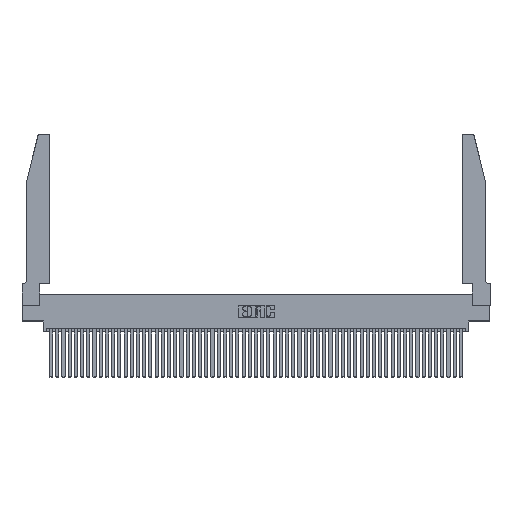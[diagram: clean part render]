
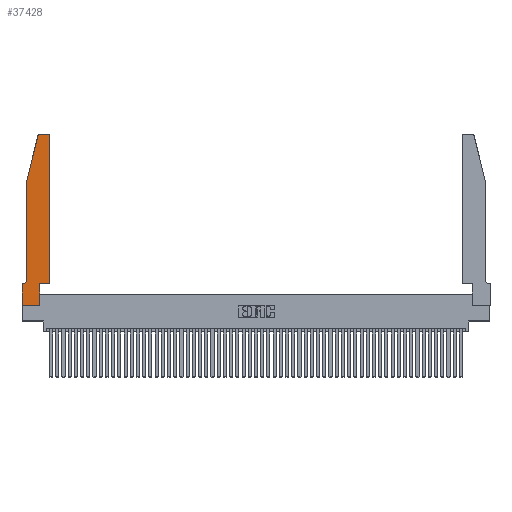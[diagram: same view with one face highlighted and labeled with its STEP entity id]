
A CAD part, top view. The second image highlights one B-rep face of the part: STEP entity #37428.
In plain terms, the highlighted planar face has unit normal (0, 0, 1).
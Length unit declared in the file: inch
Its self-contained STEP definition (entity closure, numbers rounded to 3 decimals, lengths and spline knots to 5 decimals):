
#1467 = VERTEX_POINT ( 'NONE', #30838 ) ;
#4908 = VECTOR ( 'NONE', #38754, 39.37008 ) ;
#5191 = ORIENTED_EDGE ( 'NONE', *, *, #21473, .T. ) ;
#6381 = LINE ( 'NONE', #33834, #38349 ) ;
#10282 = VECTOR ( 'NONE', #19206, 39.37008 ) ;
#10430 = VECTOR ( 'NONE', #53533, 39.37008 ) ;
#10548 = CARTESIAN_POINT ( 'NONE',  ( 0.4205, 2.72, 0.37 ) ) ;
#10825 = CARTESIAN_POINT ( 'NONE',  ( 0.0755, 0.42, 0.37 ) ) ;
#11624 = LINE ( 'NONE', #31659, #10282 ) ;
#11645 = FACE_OUTER_BOUND ( 'NONE', #47028, .T. ) ;
#11831 = ORIENTED_EDGE ( 'NONE', *, *, #52363, .T. ) ;
#12382 = DIRECTION ( 'NONE',  ( 0., 1., 0. ) ) ;
#12933 = VERTEX_POINT ( 'NONE', #28234 ) ;
#13302 = DIRECTION ( 'NONE',  ( 0., -1., 0. ) ) ;
#13652 = LINE ( 'NONE', #20702, #53766 ) ;
#13693 = EDGE_CURVE ( 'NONE', #47984, #1467, #21667, .T. ) ;
#14218 = AXIS2_PLACEMENT_3D ( 'NONE', #49524, #24896, #53677 ) ;
#14464 = CIRCLE ( 'NONE', #14218, 0.03 ) ;
#14589 = CARTESIAN_POINT ( 'NONE',  ( 0.2605, 2.75, 0.37 ) ) ;
#14800 = DIRECTION ( 'NONE',  ( 1., 0., 0. ) ) ;
#15106 = ORIENTED_EDGE ( 'NONE', *, *, #33840, .T. ) ;
#15964 = VECTOR ( 'NONE', #13302, 39.37008 ) ;
#18115 = ORIENTED_EDGE ( 'NONE', *, *, #38437, .T. ) ;
#18135 = CARTESIAN_POINT ( 'NONE',  ( 0.4505, 0.35, 0.37 ) ) ;
#18315 = ORIENTED_EDGE ( 'NONE', *, *, #13693, .T. ) ;
#19206 = DIRECTION ( 'NONE',  ( 1., 0., 0. ) ) ;
#19748 = PLANE ( 'NONE',  #32671 ) ;
#19885 = ORIENTED_EDGE ( 'NONE', *, *, #25951, .T. ) ;
#20147 = CARTESIAN_POINT ( 'NONE',  ( 0.25487, 2.72718, 0.37 ) ) ;
#20403 = DIRECTION ( 'NONE',  ( 0., 0., -1. ) ) ;
#20702 = CARTESIAN_POINT ( 'NONE',  ( 0.2865, 0.35, 0.37 ) ) ;
#20800 = VERTEX_POINT ( 'NONE', #34081 ) ;
#20830 = CIRCLE ( 'NONE', #30620, 0.07 ) ;
#20888 = CARTESIAN_POINT ( 'NONE',  ( 0.2865, 0., 0.37 ) ) ;
#21217 = VERTEX_POINT ( 'NONE', #20147 ) ;
#21420 = CARTESIAN_POINT ( 'NONE',  ( 0.2865, 0.35, 0.37 ) ) ;
#21473 = EDGE_CURVE ( 'NONE', #48769, #26738, #31640, .T. ) ;
#21660 = VERTEX_POINT ( 'NONE', #46624 ) ;
#21667 = LINE ( 'NONE', #33025, #10430 ) ;
#21725 = VECTOR ( 'NONE', #39441, 39.37008 ) ;
#22203 = ORIENTED_EDGE ( 'NONE', *, *, #53628, .T. ) ;
#22237 = VECTOR ( 'NONE', #51104, 39.37008 ) ;
#22417 = AXIS2_PLACEMENT_3D ( 'NONE', #10548, #39639, #14800 ) ;
#23539 = CARTESIAN_POINT ( 'NONE',  ( 0.0055, 0.35, 0.37 ) ) ;
#23729 = EDGE_CURVE ( 'NONE', #30649, #20800, #51973, .T. ) ;
#24896 = DIRECTION ( 'NONE',  ( 0., 0., 1. ) ) ;
#25675 = ORIENTED_EDGE ( 'NONE', *, *, #38098, .T. ) ;
#25825 = CARTESIAN_POINT ( 'NONE',  ( 0.4505, 0.35, 0.37 ) ) ;
#25886 = CARTESIAN_POINT ( 'NONE',  ( 0.4505, 0.35, 0.37 ) ) ;
#25951 = EDGE_CURVE ( 'NONE', #33704, #35712, #13652, .T. ) ;
#26738 = VERTEX_POINT ( 'NONE', #50830 ) ;
#27995 = ORIENTED_EDGE ( 'NONE', *, *, #37023, .T. ) ;
#28037 = DIRECTION ( 'NONE',  ( 1., 0., 0. ) ) ;
#28234 = CARTESIAN_POINT ( 'NONE',  ( 0.0755, 2., 0.37 ) ) ;
#28399 = EDGE_CURVE ( 'NONE', #20800, #21217, #14464, .T. ) ;
#29688 = CARTESIAN_POINT ( 'NONE',  ( 0., 0., 0.37 ) ) ;
#30040 = DIRECTION ( 'NONE',  ( 0., 1., 0. ) ) ;
#30351 = VECTOR ( 'NONE', #30040, 39.37008 ) ;
#30620 = AXIS2_PLACEMENT_3D ( 'NONE', #45053, #20403, #49195 ) ;
#30649 = VERTEX_POINT ( 'NONE', #31062 ) ;
#30838 = CARTESIAN_POINT ( 'NONE',  ( 0., 0.35, 0.37 ) ) ;
#31062 = CARTESIAN_POINT ( 'NONE',  ( 0.4205, 2.75, 0.37 ) ) ;
#31640 = LINE ( 'NONE', #25886, #30351 ) ;
#31659 = CARTESIAN_POINT ( 'NONE',  ( 0., 0., 0.37 ) ) ;
#32671 = AXIS2_PLACEMENT_3D ( 'NONE', #48544, #52675, #28037 ) ;
#33025 = CARTESIAN_POINT ( 'NONE',  ( 0.0755, 0.35, 0.37 ) ) ;
#33181 = ORIENTED_EDGE ( 'NONE', *, *, #23729, .T. ) ;
#33187 = LINE ( 'NONE', #18135, #22237 ) ;
#33704 = VERTEX_POINT ( 'NONE', #20888 ) ;
#33834 = CARTESIAN_POINT ( 'NONE',  ( 0.0755, 2., 0.37 ) ) ;
#33840 = EDGE_CURVE ( 'NONE', #1467, #21660, #48914, .T. ) ;
#34081 = CARTESIAN_POINT ( 'NONE',  ( 0.284, 2.75, 0.37 ) ) ;
#35712 = VERTEX_POINT ( 'NONE', #21420 ) ;
#37023 = EDGE_CURVE ( 'NONE', #12933, #51143, #6381, .T. ) ;
#37428 = ADVANCED_FACE ( 'NONE', ( #11645 ), #19748, .T. ) ;
#37979 = DIRECTION ( 'NONE',  ( 0., -1., 0. ) ) ;
#38098 = EDGE_CURVE ( 'NONE', #51143, #47984, #20830, .T. ) ;
#38307 = ORIENTED_EDGE ( 'NONE', *, *, #41718, .T. ) ;
#38349 = VECTOR ( 'NONE', #37979, 39.37008 ) ;
#38437 = EDGE_CURVE ( 'NONE', #21217, #12933, #49128, .T. ) ;
#38754 = DIRECTION ( 'NONE',  ( -0.239, -0.971, 0. ) ) ;
#39441 = DIRECTION ( 'NONE',  ( -1., 0., 0. ) ) ;
#39639 = DIRECTION ( 'NONE',  ( 0., 0., 1. ) ) ;
#39841 = CIRCLE ( 'NONE', #22417, 0.03 ) ;
#41718 = EDGE_CURVE ( 'NONE', #35712, #48769, #33187, .T. ) ;
#45053 = CARTESIAN_POINT ( 'NONE',  ( 0.0055, 0.42, 0.37 ) ) ;
#45960 = ORIENTED_EDGE ( 'NONE', *, *, #28399, .T. ) ;
#46624 = CARTESIAN_POINT ( 'NONE',  ( 0., 0., 0.37 ) ) ;
#46826 = CARTESIAN_POINT ( 'NONE',  ( 0.0755, 2., 0.37 ) ) ;
#47028 = EDGE_LOOP ( 'NONE', ( #33181, #45960, #18115, #27995, #25675, #18315, #15106, #22203, #19885, #38307, #5191, #11831 ) ) ;
#47984 = VERTEX_POINT ( 'NONE', #23539 ) ;
#48544 = CARTESIAN_POINT ( 'NONE',  ( 0., 0.35, 0.37 ) ) ;
#48769 = VERTEX_POINT ( 'NONE', #25825 ) ;
#48914 = LINE ( 'NONE', #29688, #15964 ) ;
#49128 = LINE ( 'NONE', #46826, #4908 ) ;
#49195 = DIRECTION ( 'NONE',  ( -1., 0., 0. ) ) ;
#49524 = CARTESIAN_POINT ( 'NONE',  ( 0.284, 2.72, 0.37 ) ) ;
#50830 = CARTESIAN_POINT ( 'NONE',  ( 0.4505, 2.72, 0.37 ) ) ;
#51104 = DIRECTION ( 'NONE',  ( 1., 0., 0. ) ) ;
#51143 = VERTEX_POINT ( 'NONE', #10825 ) ;
#51973 = LINE ( 'NONE', #14589, #21725 ) ;
#52363 = EDGE_CURVE ( 'NONE', #26738, #30649, #39841, .T. ) ;
#52675 = DIRECTION ( 'NONE',  ( 0., 0., 1. ) ) ;
#53533 = DIRECTION ( 'NONE',  ( -1., 0., 0. ) ) ;
#53628 = EDGE_CURVE ( 'NONE', #21660, #33704, #11624, .T. ) ;
#53677 = DIRECTION ( 'NONE',  ( 1., 0., 0. ) ) ;
#53766 = VECTOR ( 'NONE', #12382, 39.37008 ) ;
